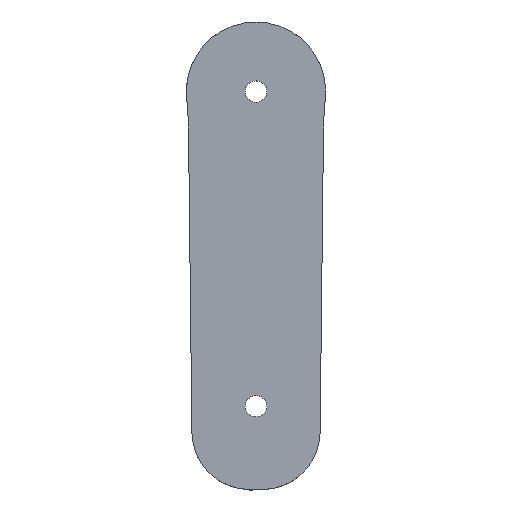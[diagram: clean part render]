
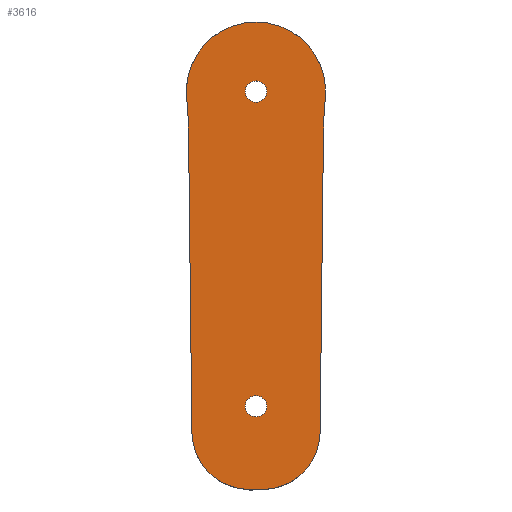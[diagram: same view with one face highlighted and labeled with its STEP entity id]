
A CAD part, top view. The second image highlights one B-rep face of the part: STEP entity #3616.
In plain terms, the highlighted planar face has unit normal (0, 0, 1).
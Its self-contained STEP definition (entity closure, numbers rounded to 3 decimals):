
#228=FACE_BOUND('',#433,.T.);
#229=FACE_BOUND('',#434,.T.);
#234=FACE_OUTER_BOUND('',#432,.T.);
#432=EDGE_LOOP('',(#2337,#2338,#2339,#2340,#2341,#2342,#2343,#2344));
#433=EDGE_LOOP('',(#2345));
#434=EDGE_LOOP('',(#2346));
#636=LINE('',#5137,#970);
#637=LINE('',#5144,#971);
#970=VECTOR('',#4159,10.);
#971=VECTOR('',#4166,10.);
#1304=CIRCLE('',#3829,15.);
#1305=CIRCLE('',#3830,21.717);
#1306=CIRCLE('',#3831,15.);
#1307=CIRCLE('',#3832,100.);
#1308=CIRCLE('',#3833,17.99);
#1309=CIRCLE('',#3834,100.);
#1310=CIRCLE('',#3835,2.75);
#1311=CIRCLE('',#3836,2.75);
#1389=VERTEX_POINT('',#5129);
#1390=VERTEX_POINT('',#5130);
#1391=VERTEX_POINT('',#5132);
#1392=VERTEX_POINT('',#5134);
#1393=VERTEX_POINT('',#5136);
#1394=VERTEX_POINT('',#5138);
#1395=VERTEX_POINT('',#5140);
#1396=VERTEX_POINT('',#5142);
#1397=VERTEX_POINT('',#5145);
#1398=VERTEX_POINT('',#5147);
#1766=EDGE_CURVE('',#1389,#1390,#1304,.T.);
#1767=EDGE_CURVE('',#1391,#1389,#1305,.T.);
#1768=EDGE_CURVE('',#1392,#1391,#1306,.T.);
#1769=EDGE_CURVE('',#1393,#1392,#636,.T.);
#1770=EDGE_CURVE('',#1394,#1393,#1307,.T.);
#1771=EDGE_CURVE('',#1395,#1394,#1308,.T.);
#1772=EDGE_CURVE('',#1396,#1395,#1309,.T.);
#1773=EDGE_CURVE('',#1390,#1396,#637,.T.);
#1774=EDGE_CURVE('',#1397,#1397,#1310,.T.);
#1775=EDGE_CURVE('',#1398,#1398,#1311,.T.);
#2337=ORIENTED_EDGE('',*,*,#1766,.F.);
#2338=ORIENTED_EDGE('',*,*,#1767,.F.);
#2339=ORIENTED_EDGE('',*,*,#1768,.F.);
#2340=ORIENTED_EDGE('',*,*,#1769,.F.);
#2341=ORIENTED_EDGE('',*,*,#1770,.F.);
#2342=ORIENTED_EDGE('',*,*,#1771,.F.);
#2343=ORIENTED_EDGE('',*,*,#1772,.F.);
#2344=ORIENTED_EDGE('',*,*,#1773,.F.);
#2345=ORIENTED_EDGE('',*,*,#1774,.F.);
#2346=ORIENTED_EDGE('',*,*,#1775,.F.);
#3479=PLANE('',#3828);
#3616=ADVANCED_FACE('',(#234,#228,#229),#3479,.T.);
#3828=AXIS2_PLACEMENT_3D('',#5128,#4151,#4152);
#3829=AXIS2_PLACEMENT_3D('',#5131,#4153,#4154);
#3830=AXIS2_PLACEMENT_3D('',#5133,#4155,#4156);
#3831=AXIS2_PLACEMENT_3D('',#5135,#4157,#4158);
#3832=AXIS2_PLACEMENT_3D('',#5139,#4160,#4161);
#3833=AXIS2_PLACEMENT_3D('',#5141,#4162,#4163);
#3834=AXIS2_PLACEMENT_3D('',#5143,#4164,#4165);
#3835=AXIS2_PLACEMENT_3D('',#5146,#4167,#4168);
#3836=AXIS2_PLACEMENT_3D('',#5148,#4169,#4170);
#4151=DIRECTION('center_axis',(0.,0.,1.));
#4152=DIRECTION('ref_axis',(1.,0.,0.));
#4153=DIRECTION('center_axis',(0.,0.,-1.));
#4154=DIRECTION('ref_axis',(-0.782,-0.623,0.));
#4155=DIRECTION('center_axis',(0.,0.,-1.));
#4156=DIRECTION('ref_axis',(-1.,0.,0.));
#4157=DIRECTION('center_axis',(0.,0.,-1.));
#4158=DIRECTION('ref_axis',(0.782,-0.623,0.));
#4159=DIRECTION('',(-0.011,-1.,0.));
#4160=DIRECTION('center_axis',(0.,0.,1.));
#4161=DIRECTION('ref_axis',(-0.999,0.055,0.));
#4162=DIRECTION('center_axis',(0.,0.,-1.));
#4163=DIRECTION('ref_axis',(-0.917,0.4,0.));
#4164=DIRECTION('center_axis',(0.,0.,1.));
#4165=DIRECTION('ref_axis',(0.999,0.055,0.));
#4166=DIRECTION('',(-0.011,1.,0.));
#4167=DIRECTION('center_axis',(0.,0.,1.));
#4168=DIRECTION('ref_axis',(1.,0.,0.));
#4169=DIRECTION('center_axis',(0.,0.,1.));
#4170=DIRECTION('ref_axis',(1.,0.,0.));
#5128=CARTESIAN_POINT('Origin',(0.,-17.103,7.46));
#5129=CARTESIAN_POINT('',(-5.086,-76.993,7.46));
#5130=CARTESIAN_POINT('',(-16.572,-62.576,7.46));
#5131=CARTESIAN_POINT('Origin',(-1.573,-62.41,7.46));
#5132=CARTESIAN_POINT('',(5.086,-76.993,7.46));
#5133=CARTESIAN_POINT('Origin',(0.,-55.88,7.46));
#5134=CARTESIAN_POINT('',(16.572,-62.576,7.46));
#5135=CARTESIAN_POINT('Origin',(1.573,-62.41,7.46));
#5136=CARTESIAN_POINT('',(17.428,14.941,7.46));
#5137=CARTESIAN_POINT('',(17.329,5.951,7.46));
#5138=CARTESIAN_POINT('',(17.903,23.637,7.46));
#5139=CARTESIAN_POINT('Origin',(117.422,13.837,7.46));
#5140=CARTESIAN_POINT('',(-17.903,23.637,7.46));
#5141=CARTESIAN_POINT('Origin',(0.,25.4,7.46));
#5142=CARTESIAN_POINT('',(-17.428,14.941,7.46));
#5143=CARTESIAN_POINT('Origin',(-117.422,13.837,7.46));
#5144=CARTESIAN_POINT('',(-16.781,-43.652,7.46));
#5145=CARTESIAN_POINT('',(-2.75,25.4,7.46));
#5146=CARTESIAN_POINT('Origin',(0.,25.4,7.46));
#5147=CARTESIAN_POINT('',(-2.75,-55.88,7.46));
#5148=CARTESIAN_POINT('Origin',(0.,-55.88,7.46));
